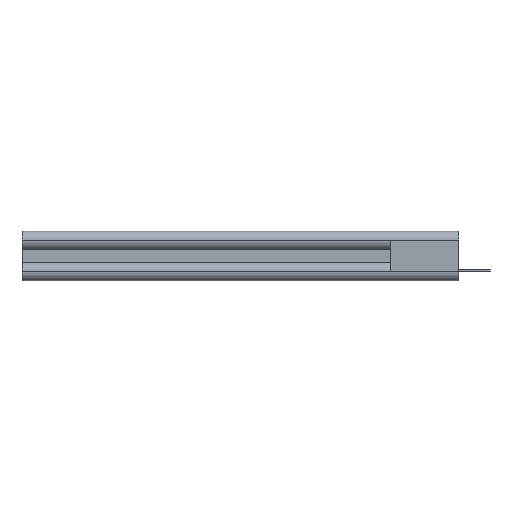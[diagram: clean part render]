
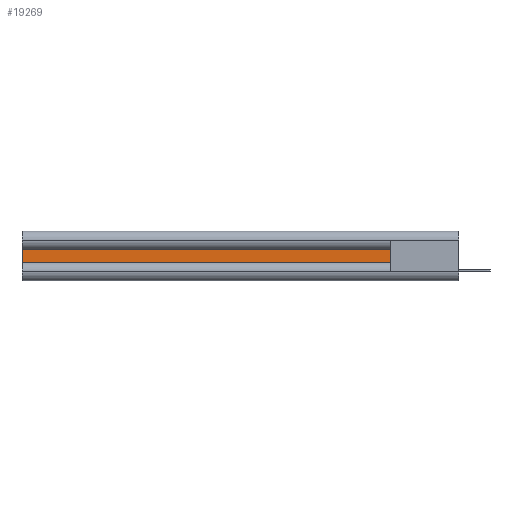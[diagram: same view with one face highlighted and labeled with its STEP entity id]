
A CAD part, left-side view. The second image highlights one B-rep face of the part: STEP entity #19269.
In plain terms, the highlighted planar face has unit normal (-1, 0, 0).
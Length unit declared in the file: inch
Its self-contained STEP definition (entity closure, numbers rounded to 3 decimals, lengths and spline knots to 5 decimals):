
#275 = ORIENTED_EDGE ( 'NONE', *, *, #19650, .T. ) ;
#706 = VERTEX_POINT ( 'NONE', #20007 ) ;
#1277 = DIRECTION ( 'NONE',  ( 0., 0., -1. ) ) ;
#2113 = EDGE_LOOP ( 'NONE', ( #275, #3665, #13271, #9270 ) ) ;
#3037 = EDGE_CURVE ( 'NONE', #6999, #19013, #12815, .T. ) ;
#3120 = DIRECTION ( 'NONE',  ( 0., 0., -1. ) ) ;
#3665 = ORIENTED_EDGE ( 'NONE', *, *, #20350, .T. ) ;
#5917 = EDGE_CURVE ( 'NONE', #6199, #6999, #10648, .T. ) ;
#6199 = VERTEX_POINT ( 'NONE', #15857 ) ;
#6794 = CARTESIAN_POINT ( 'NONE',  ( 0.044, 3., -0.0465 ) ) ;
#6881 = AXIS2_PLACEMENT_3D ( 'NONE', #22821, #12278, #1277 ) ;
#6999 = VERTEX_POINT ( 'NONE', #9239 ) ;
#7564 = LINE ( 'NONE', #6794, #16671 ) ;
#8579 = PLANE ( 'NONE',  #6881 ) ;
#9239 = CARTESIAN_POINT ( 'NONE',  ( 0.044, 0.473, -0.0465 ) ) ;
#9270 = ORIENTED_EDGE ( 'NONE', *, *, #5917, .F. ) ;
#9555 = FACE_OUTER_BOUND ( 'NONE', #2113, .T. ) ;
#9903 = CARTESIAN_POINT ( 'NONE',  ( 0.044, 0.37012, 0.0465 ) ) ;
#10648 = LINE ( 'NONE', #20902, #19112 ) ;
#12278 = DIRECTION ( 'NONE',  ( 1., 0., 0. ) ) ;
#12815 = LINE ( 'NONE', #18039, #17035 ) ;
#13217 = CARTESIAN_POINT ( 'NONE',  ( 0.044, 3., -0.0465 ) ) ;
#13271 = ORIENTED_EDGE ( 'NONE', *, *, #3037, .F. ) ;
#15398 = DIRECTION ( 'NONE',  ( 0., 1., 0. ) ) ;
#15498 = LINE ( 'NONE', #9903, #19686 ) ;
#15857 = CARTESIAN_POINT ( 'NONE',  ( 0.044, 0.473, 0.0465 ) ) ;
#16671 = VECTOR ( 'NONE', #3120, 39.37008 ) ;
#17035 = VECTOR ( 'NONE', #18383, 39.37008 ) ;
#18039 = CARTESIAN_POINT ( 'NONE',  ( 0.044, 0.37012, -0.0465 ) ) ;
#18383 = DIRECTION ( 'NONE',  ( 0., 1., 0. ) ) ;
#19013 = VERTEX_POINT ( 'NONE', #13217 ) ;
#19112 = VECTOR ( 'NONE', #20721, 39.37008 ) ;
#19269 = ADVANCED_FACE ( 'NONE', ( #9555 ), #8579, .F. ) ;
#19650 = EDGE_CURVE ( 'NONE', #6199, #706, #15498, .T. ) ;
#19686 = VECTOR ( 'NONE', #15398, 39.37008 ) ;
#20007 = CARTESIAN_POINT ( 'NONE',  ( 0.044, 3., 0.0465 ) ) ;
#20350 = EDGE_CURVE ( 'NONE', #706, #19013, #7564, .T. ) ;
#20721 = DIRECTION ( 'NONE',  ( 0., 0., -1. ) ) ;
#20902 = CARTESIAN_POINT ( 'NONE',  ( 0.044, 0.473, -0.0465 ) ) ;
#22821 = CARTESIAN_POINT ( 'NONE',  ( 0.044, 0.37012, -0.0465 ) ) ;
